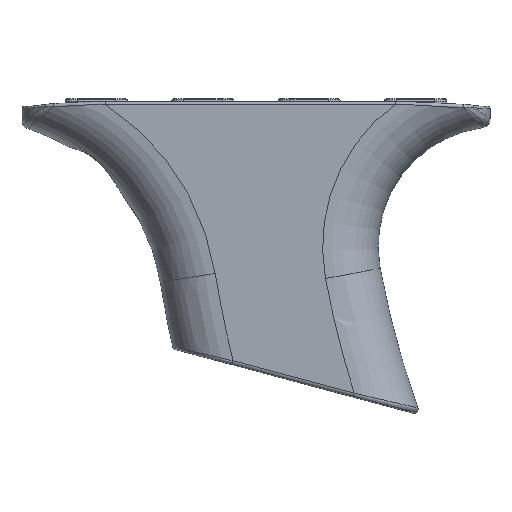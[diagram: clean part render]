
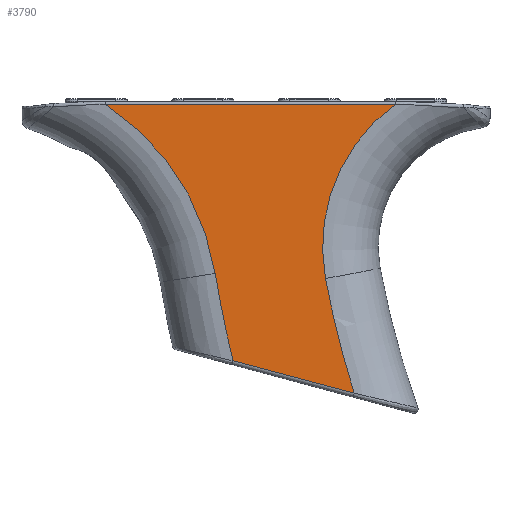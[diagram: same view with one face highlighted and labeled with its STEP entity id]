
A CAD part, left-side view. The second image highlights one B-rep face of the part: STEP entity #3790.
In plain terms, the highlighted planar face has unit normal (-1, 0, 0).
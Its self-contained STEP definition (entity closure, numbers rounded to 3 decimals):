
#251=PLANE('',#4132);
#458=FACE_OUTER_BOUND('',#724,.T.);
#724=EDGE_LOOP('',(#2951,#2952,#2953,#2954,#2955,#2956));
#994=LINE('',#7382,#1212);
#1000=LINE('',#7569,#1218);
#1212=VECTOR('',#4782,10.);
#1218=VECTOR('',#4842,11.);
#1442=CIRCLE('',#4126,198.);
#1447=CIRCLE('',#4133,177.731);
#1448=CIRCLE('',#4134,33.);
#1449=CIRCLE('',#4135,46.75);
#1775=VERTEX_POINT('',#7368);
#1777=VERTEX_POINT('',#7380);
#1787=VERTEX_POINT('',#7555);
#1789=VERTEX_POINT('',#7564);
#1790=VERTEX_POINT('',#7566);
#1791=VERTEX_POINT('',#7568);
#2182=EDGE_CURVE('',#1777,#1775,#994,.T.);
#2202=EDGE_CURVE('',#1787,#1775,#1442,.T.);
#2207=EDGE_CURVE('',#1777,#1789,#1447,.T.);
#2208=EDGE_CURVE('',#1789,#1790,#1448,.T.);
#2209=EDGE_CURVE('',#1791,#1790,#1000,.T.);
#2210=EDGE_CURVE('',#1787,#1791,#1449,.T.);
#2951=ORIENTED_EDGE('',*,*,#2182,.F.);
#2952=ORIENTED_EDGE('',*,*,#2207,.T.);
#2953=ORIENTED_EDGE('',*,*,#2208,.T.);
#2954=ORIENTED_EDGE('',*,*,#2209,.F.);
#2955=ORIENTED_EDGE('',*,*,#2210,.F.);
#2956=ORIENTED_EDGE('',*,*,#2202,.T.);
#3790=ADVANCED_FACE('',(#458),#251,.T.);
#4126=AXIS2_PLACEMENT_3D('',#7556,#4824,#4825);
#4132=AXIS2_PLACEMENT_3D('',#7563,#4836,#4837);
#4133=AXIS2_PLACEMENT_3D('',#7565,#4838,#4839);
#4134=AXIS2_PLACEMENT_3D('',#7567,#4840,#4841);
#4135=AXIS2_PLACEMENT_3D('',#7570,#4843,#4844);
#4782=DIRECTION('',(0.,0.966,0.259));
#4824=DIRECTION('center_axis',(-1.,0.,0.));
#4825=DIRECTION('ref_axis',(0.,0.965,-0.26));
#4836=DIRECTION('center_axis',(-1.,0.,0.));
#4837=DIRECTION('ref_axis',(0.,-1.,0.));
#4838=DIRECTION('center_axis',(1.,0.,0.));
#4839=DIRECTION('ref_axis',(0.,0.957,-0.289));
#4840=DIRECTION('center_axis',(1.,0.,0.));
#4841=DIRECTION('ref_axis',(0.,0.915,0.402));
#4842=DIRECTION('',(0.,-1.,0.));
#4843=DIRECTION('center_axis',(-1.,0.,0.));
#4844=DIRECTION('ref_axis',(0.,0.,
-1.));
#7368=CARTESIAN_POINT('',(-11.75,-119.796,55.186));
#7380=CARTESIAN_POINT('',(-11.75,-142.581,49.089));
#7382=CARTESIAN_POINT('',(-11.75,-197.912,34.282));
#7555=CARTESIAN_POINT('',(-11.75,-116.435,71.634));
#7556=CARTESIAN_POINT('Origin',(-11.75,-311.932,103.019));
#7563=CARTESIAN_POINT('Origin',(-11.75,-300.939,103.019));
#7564=CARTESIAN_POINT('',(-11.75,-137.171,70.663));
#7565=CARTESIAN_POINT('Origin',(-11.75,-311.932,103.019));
#7566=CARTESIAN_POINT('',(-11.75,-150.309,103.431));
#7567=CARTESIAN_POINT('Origin',(-11.75,-169.62,76.67));
#7568=CARTESIAN_POINT('',(-11.75,-95.74,103.431));
#7569=CARTESIAN_POINT('',(-11.75,-80.101,103.431));
#7570=CARTESIAN_POINT('Origin',(-11.75,-70.276,64.224));
